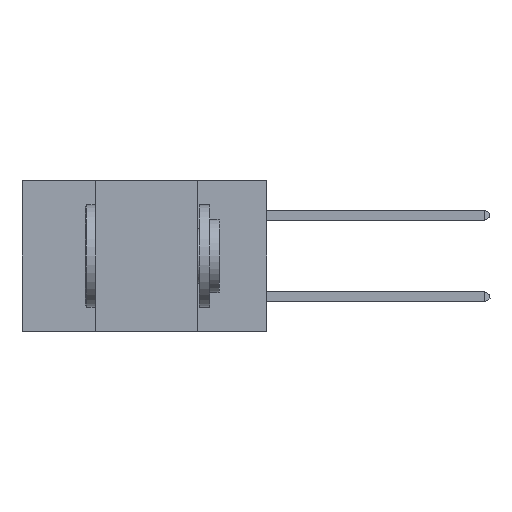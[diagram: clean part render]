
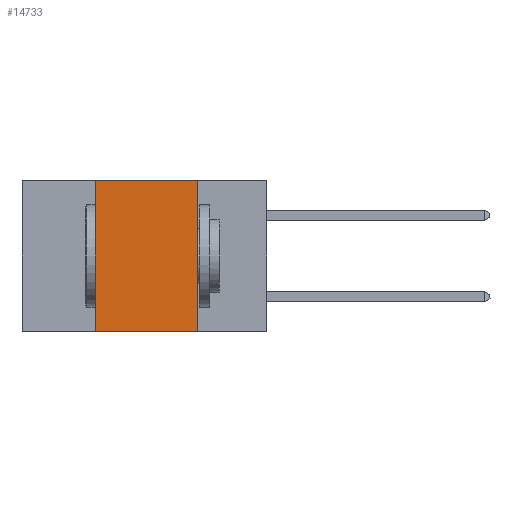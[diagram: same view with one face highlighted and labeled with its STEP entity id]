
A CAD part, left-side view. The second image highlights one B-rep face of the part: STEP entity #14733.
In plain terms, the highlighted planar face has unit normal (-1, 0, 0).
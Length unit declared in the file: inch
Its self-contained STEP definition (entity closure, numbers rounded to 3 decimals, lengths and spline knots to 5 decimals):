
#344 = VECTOR ( 'NONE', #10200, 39.37008 ) ;
#1307 = CARTESIAN_POINT ( 'NONE',  ( 0., 0.6, -0.37 ) ) ;
#1833 = CARTESIAN_POINT ( 'NONE',  ( 0., 0.6, 0. ) ) ;
#2033 = DIRECTION ( 'NONE',  ( 0., -1., 0. ) ) ;
#3383 = DIRECTION ( 'NONE',  ( 0., 0., -1. ) ) ;
#4344 = LINE ( 'NONE', #1307, #344 ) ;
#4375 = DIRECTION ( 'NONE',  ( 0., 0., -1. ) ) ;
#5167 = DIRECTION ( 'NONE',  ( 0., 0., 1. ) ) ;
#5242 = EDGE_CURVE ( 'NONE', #14552, #16586, #4344, .T. ) ;
#5618 = CARTESIAN_POINT ( 'NONE',  ( 0., 0.17, 0. ) ) ;
#6211 = EDGE_CURVE ( 'NONE', #14552, #12404, #14580, .T. ) ;
#6735 = LINE ( 'NONE', #14585, #17340 ) ;
#7355 = CARTESIAN_POINT ( 'NONE',  ( 0., 0.42, -0.37 ) ) ;
#7455 = ORIENTED_EDGE ( 'NONE', *, *, #9194, .F. ) ;
#7708 = ORIENTED_EDGE ( 'NONE', *, *, #17925, .F. ) ;
#8073 = LINE ( 'NONE', #9426, #15292 ) ;
#8281 = ORIENTED_EDGE ( 'NONE', *, *, #6211, .F. ) ;
#9194 = EDGE_CURVE ( 'NONE', #18231, #16586, #6735, .T. ) ;
#9426 = CARTESIAN_POINT ( 'NONE',  ( 0., 0.6, 0. ) ) ;
#9527 = ORIENTED_EDGE ( 'NONE', *, *, #5242, .T. ) ;
#9938 = AXIS2_PLACEMENT_3D ( 'NONE', #1833, #12216, #3383 ) ;
#10200 = DIRECTION ( 'NONE',  ( 0., -1., 0. ) ) ;
#10643 = EDGE_LOOP ( 'NONE', ( #7455, #7708, #8281, #9527 ) ) ;
#10804 = VECTOR ( 'NONE', #5167, 39.37008 ) ;
#12216 = DIRECTION ( 'NONE',  ( 1., 0., 0. ) ) ;
#12404 = VERTEX_POINT ( 'NONE', #13882 ) ;
#13424 = FACE_OUTER_BOUND ( 'NONE', #10643, .T. ) ;
#13882 = CARTESIAN_POINT ( 'NONE',  ( 0., 0.42, 0. ) ) ;
#14552 = VERTEX_POINT ( 'NONE', #7355 ) ;
#14580 = LINE ( 'NONE', #18056, #10804 ) ;
#14585 = CARTESIAN_POINT ( 'NONE',  ( 0., 0.17, 0. ) ) ;
#14733 = ADVANCED_FACE ( 'NONE', ( #13424 ), #14954, .F. ) ;
#14954 = PLANE ( 'NONE',  #9938 ) ;
#15292 = VECTOR ( 'NONE', #2033, 39.37008 ) ;
#16586 = VERTEX_POINT ( 'NONE', #18736 ) ;
#17340 = VECTOR ( 'NONE', #4375, 39.37008 ) ;
#17925 = EDGE_CURVE ( 'NONE', #12404, #18231, #8073, .T. ) ;
#18056 = CARTESIAN_POINT ( 'NONE',  ( 0., 0.42, 0. ) ) ;
#18231 = VERTEX_POINT ( 'NONE', #5618 ) ;
#18736 = CARTESIAN_POINT ( 'NONE',  ( 0., 0.17, -0.37 ) ) ;
